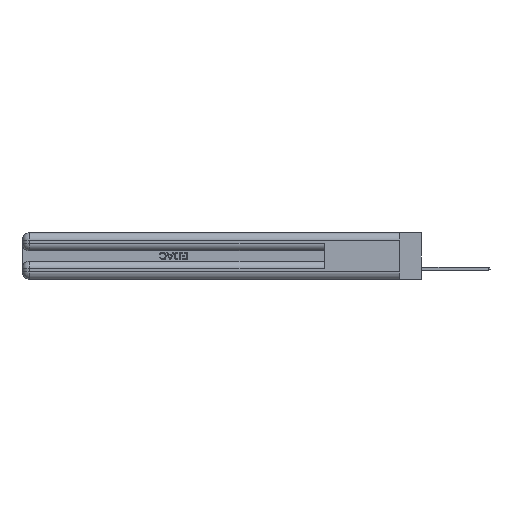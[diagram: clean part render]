
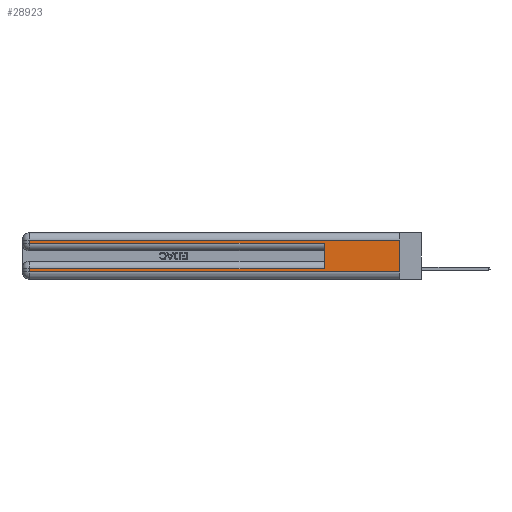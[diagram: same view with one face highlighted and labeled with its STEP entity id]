
A CAD part, left-side view. The second image highlights one B-rep face of the part: STEP entity #28923.
In plain terms, the highlighted planar face has unit normal (-1, 0, 0).
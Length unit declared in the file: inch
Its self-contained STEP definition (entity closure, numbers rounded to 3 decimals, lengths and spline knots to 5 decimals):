
#6 = VECTOR ( 'NONE', #540, 39.37008 ) ;
#540 = DIRECTION ( 'NONE',  ( 0., -1., 0. ) ) ;
#595 = CARTESIAN_POINT ( 'NONE',  ( 0., 0., 0.37 ) ) ;
#638 = FACE_OUTER_BOUND ( 'NONE', #43292, .T. ) ;
#737 = VECTOR ( 'NONE', #39427, 39.37008 ) ;
#794 = DIRECTION ( 'NONE',  ( 0., -1., 0. ) ) ;
#1022 = CARTESIAN_POINT ( 'NONE',  ( 0., 0., 0.285 ) ) ;
#1095 = VECTOR ( 'NONE', #36505, 39.37008 ) ;
#1222 = VECTOR ( 'NONE', #45465, 39.37008 ) ;
#1680 = DIRECTION ( 'NONE',  ( 0., 1., 0. ) ) ;
#2032 = EDGE_CURVE ( 'NONE', #29193, #10314, #30772, .T. ) ;
#2287 = CARTESIAN_POINT ( 'NONE',  ( 0., 0., 0.37 ) ) ;
#2358 = ORIENTED_EDGE ( 'NONE', *, *, #2032, .T. ) ;
#2699 = VECTOR ( 'NONE', #43332, 39.37008 ) ;
#2896 = CARTESIAN_POINT ( 'NONE',  ( 0., 0.6, 0.085 ) ) ;
#3164 = CARTESIAN_POINT ( 'NONE',  ( 0., 0., 0.06 ) ) ;
#3181 = VECTOR ( 'NONE', #794, 39.37008 ) ;
#3626 = EDGE_CURVE ( 'NONE', #10314, #46204, #9917, .T. ) ;
#4733 = CARTESIAN_POINT ( 'NONE',  ( 0., 2.94, 0.085 ) ) ;
#5548 = CARTESIAN_POINT ( 'NONE',  ( 0., 2.94, 0.06 ) ) ;
#5869 = DIRECTION ( 'NONE',  ( 0., 0., -1. ) ) ;
#6027 = EDGE_CURVE ( 'NONE', #41967, #12594, #34328, .T. ) ;
#9228 = VERTEX_POINT ( 'NONE', #22566 ) ;
#9761 = LINE ( 'NONE', #11936, #23152 ) ;
#9917 = LINE ( 'NONE', #27279, #3181 ) ;
#10314 = VERTEX_POINT ( 'NONE', #5548 ) ;
#10325 = ORIENTED_EDGE ( 'NONE', *, *, #29067, .F. ) ;
#10779 = LINE ( 'NONE', #595, #1222 ) ;
#11936 = CARTESIAN_POINT ( 'NONE',  ( 0., 2.94, 0.37 ) ) ;
#12576 = ORIENTED_EDGE ( 'NONE', *, *, #18719, .T. ) ;
#12594 = VERTEX_POINT ( 'NONE', #36606 ) ;
#13077 = ORIENTED_EDGE ( 'NONE', *, *, #6027, .F. ) ;
#13262 = VECTOR ( 'NONE', #1680, 39.37008 ) ;
#14236 = CARTESIAN_POINT ( 'NONE',  ( 0., 0., 0.31 ) ) ;
#15898 = CARTESIAN_POINT ( 'NONE',  ( 0., 0., 0.085 ) ) ;
#18719 = EDGE_CURVE ( 'NONE', #41074, #9228, #9761, .T. ) ;
#19612 = ORIENTED_EDGE ( 'NONE', *, *, #42332, .T. ) ;
#20758 = AXIS2_PLACEMENT_3D ( 'NONE', #2287, #38474, #31172 ) ;
#21274 = CARTESIAN_POINT ( 'NONE',  ( 0., 0.6, 0.145 ) ) ;
#22566 = CARTESIAN_POINT ( 'NONE',  ( 0., 2.94, 0.285 ) ) ;
#23152 = VECTOR ( 'NONE', #5869, 39.37008 ) ;
#24396 = ORIENTED_EDGE ( 'NONE', *, *, #30804, .T. ) ;
#25294 = EDGE_CURVE ( 'NONE', #31306, #41074, #33923, .T. ) ;
#27279 = CARTESIAN_POINT ( 'NONE',  ( 0., 0., 0.06 ) ) ;
#27338 = LINE ( 'NONE', #1022, #6 ) ;
#27598 = CARTESIAN_POINT ( 'NONE',  ( 0., 0., 0.31 ) ) ;
#28923 = ADVANCED_FACE ( 'NONE', ( #638 ), #30537, .F. ) ;
#29067 = EDGE_CURVE ( 'NONE', #31306, #46204, #10779, .T. ) ;
#29193 = VERTEX_POINT ( 'NONE', #4733 ) ;
#30537 = PLANE ( 'NONE',  #20758 ) ;
#30751 = ORIENTED_EDGE ( 'NONE', *, *, #3626, .T. ) ;
#30772 = LINE ( 'NONE', #40230, #1095 ) ;
#30804 = EDGE_CURVE ( 'NONE', #9228, #12594, #27338, .T. ) ;
#31172 = DIRECTION ( 'NONE',  ( 0., 0., -1. ) ) ;
#31306 = VERTEX_POINT ( 'NONE', #27598 ) ;
#33923 = LINE ( 'NONE', #14236, #2699 ) ;
#34328 = LINE ( 'NONE', #21274, #737 ) ;
#36505 = DIRECTION ( 'NONE',  ( 0., 0., -1. ) ) ;
#36606 = CARTESIAN_POINT ( 'NONE',  ( 0., 0.6, 0.285 ) ) ;
#38474 = DIRECTION ( 'NONE',  ( 1., 0., 0. ) ) ;
#38862 = ORIENTED_EDGE ( 'NONE', *, *, #25294, .T. ) ;
#39427 = DIRECTION ( 'NONE',  ( 0., 0., 1. ) ) ;
#40230 = CARTESIAN_POINT ( 'NONE',  ( 0., 2.94, 0.37 ) ) ;
#41074 = VERTEX_POINT ( 'NONE', #44286 ) ;
#41165 = LINE ( 'NONE', #15898, #13262 ) ;
#41967 = VERTEX_POINT ( 'NONE', #2896 ) ;
#42332 = EDGE_CURVE ( 'NONE', #41967, #29193, #41165, .T. ) ;
#43292 = EDGE_LOOP ( 'NONE', ( #10325, #38862, #12576, #24396, #13077, #19612, #2358, #30751 ) ) ;
#43332 = DIRECTION ( 'NONE',  ( 0., 1., 0. ) ) ;
#44286 = CARTESIAN_POINT ( 'NONE',  ( 0., 2.94, 0.31 ) ) ;
#45465 = DIRECTION ( 'NONE',  ( 0., 0., -1. ) ) ;
#46204 = VERTEX_POINT ( 'NONE', #3164 ) ;
